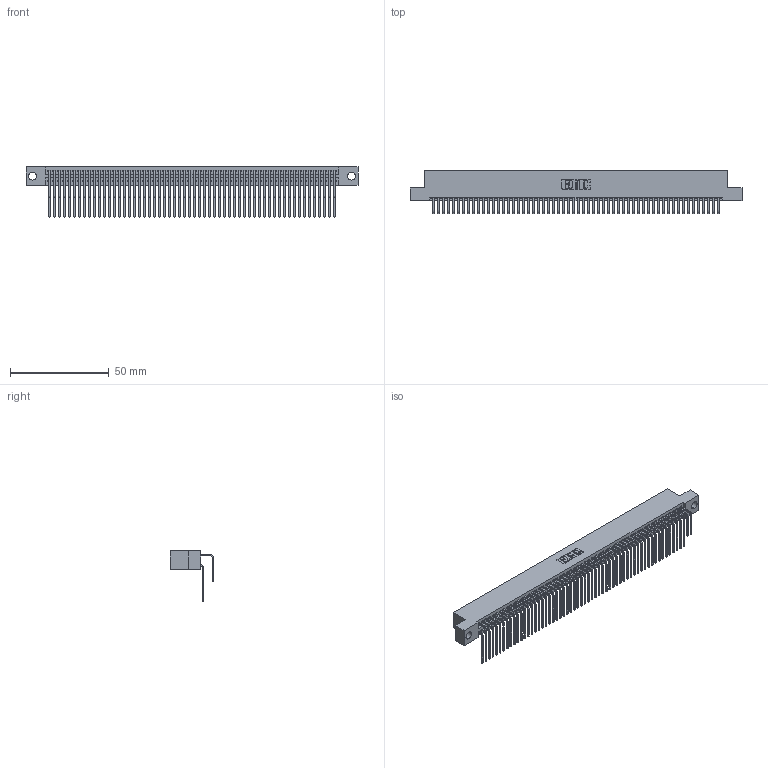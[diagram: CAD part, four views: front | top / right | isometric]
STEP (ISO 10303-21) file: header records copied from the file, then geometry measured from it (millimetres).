
FILE_DESCRIPTION (( 'STEP AP203' ), '1' );
FILE_NAME ('395-116-558-204.STEP', '2021-06-17T19:43:43', ( '' ), ( '' ), 'SwSTEP 2.0', 'SolidWorks 2020', '' );
FILE_SCHEMA (( 'CONFIG_CONTROL_DESIGN' ));
Length unit declared in the file: inch
Products named in the file (4): 345 Part_Flush Mounting Lugs - 0.156 Dia-TI; 395-116-558-204; 345-292-001_558 559 Tail - 1; 345-292-001_558 Tail - 2
Assembly tree (117 placements, depth 2):
  395-116-558-204
    345 Part_Flush Mounting Lugs - 0.156 Dia-TI
    345-292-001_558 559 Tail - 1  x58
    345-292-001_558 Tail - 2  x58
Bounding box: 168.53 x 21.83 x 25.53 mm (x, y, z)
Volume: 17082.8 mm3; surface area: 28559.4 mm2
Topology: 117 solids, 117 shells, 6172 faces, 18357 edges, 12082 vertices
Faces by surface type: plane 4154, cylinder 2018
Entity records: 45425 total; most frequent: CARTESIAN_POINT 7649, ORIENTED_EDGE 7530, DIRECTION 6697, EDGE_CURVE 3765, LINE 3361, VECTOR 3361, VERTEX_POINT 2506, AXIS2_PLACEMENT_3D 1668
